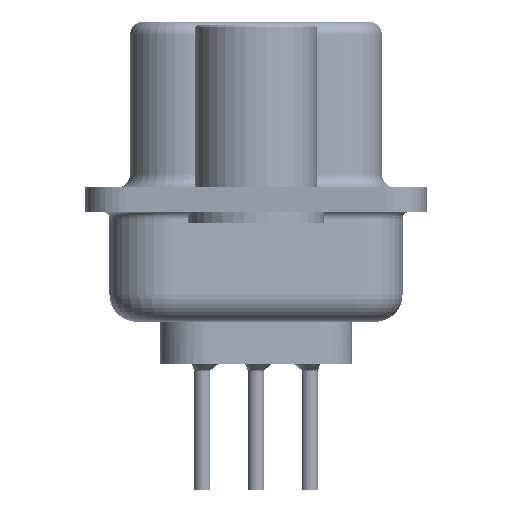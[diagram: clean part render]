
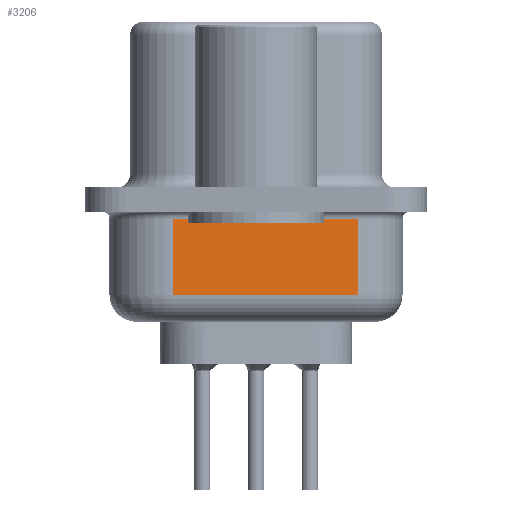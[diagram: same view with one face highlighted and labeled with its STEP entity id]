
A CAD part, left-side view. The second image highlights one B-rep face of the part: STEP entity #3206.
In plain terms, the highlighted planar face has unit normal (-0.985, -0.174, 0).
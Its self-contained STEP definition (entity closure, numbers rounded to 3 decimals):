
#273 = EDGE_CURVE ( 'NONE', #283, #12234, #12534, .T. ) ;
#283 = VERTEX_POINT ( 'NONE', #15796 ) ;
#637 = DIRECTION ( 'NONE',  ( -0.174, 0.985, 0. ) ) ;
#844 = DIRECTION ( 'NONE',  ( 0.174, -0.985, 0. ) ) ;
#3206 = ADVANCED_FACE ( 'NONE', ( #3270 ), #21578, .F. ) ;
#3270 = FACE_OUTER_BOUND ( 'NONE', #10184, .T. ) ;
#4048 = CARTESIAN_POINT ( 'NONE',  ( 3.13, 3.053, -0.7 ) ) ;
#5361 = EDGE_CURVE ( 'NONE', #12234, #35679, #33386, .T. ) ;
#8144 = VECTOR ( 'NONE', #844, 1000. ) ;
#9173 = CARTESIAN_POINT ( 'NONE',  ( 3.13, 3.053, -4.5 ) ) ;
#9586 = CARTESIAN_POINT ( 'NONE',  ( 3.13, 3.053, -3.5 ) ) ;
#10184 = EDGE_LOOP ( 'NONE', ( #37867, #31781, #35434, #33595 ) ) ;
#12234 = VERTEX_POINT ( 'NONE', #38557 ) ;
#12534 = LINE ( 'NONE', #36908, #39516 ) ;
#15191 = LINE ( 'NONE', #27587, #17185 ) ;
#15393 = DIRECTION ( 'NONE',  ( 0., 0., 1. ) ) ;
#15796 = CARTESIAN_POINT ( 'NONE',  ( 4.329, -3.747, -3.5 ) ) ;
#16301 = LINE ( 'NONE', #9586, #8144 ) ;
#17185 = VECTOR ( 'NONE', #39946, 1000. ) ;
#21578 = PLANE ( 'NONE',  #35993 ) ;
#23676 = EDGE_CURVE ( 'NONE', #25859, #283, #16301, .T. ) ;
#24268 = DIRECTION ( 'NONE',  ( -0.174, 0.985, 0. ) ) ;
#25720 = VECTOR ( 'NONE', #24268, 1000. ) ;
#25859 = VERTEX_POINT ( 'NONE', #36115 ) ;
#27587 = CARTESIAN_POINT ( 'NONE',  ( 3.13, 3.053, -4.5 ) ) ;
#27675 = DIRECTION ( 'NONE',  ( 0.985, 0.174, 0. ) ) ;
#30349 = CARTESIAN_POINT ( 'NONE',  ( 3.13, 3.053, -0.7 ) ) ;
#31781 = ORIENTED_EDGE ( 'NONE', *, *, #23676, .T. ) ;
#31963 = EDGE_CURVE ( 'NONE', #25859, #35679, #15191, .T. ) ;
#33386 = LINE ( 'NONE', #30349, #25720 ) ;
#33595 = ORIENTED_EDGE ( 'NONE', *, *, #5361, .T. ) ;
#35434 = ORIENTED_EDGE ( 'NONE', *, *, #273, .T. ) ;
#35679 = VERTEX_POINT ( 'NONE', #4048 ) ;
#35993 = AXIS2_PLACEMENT_3D ( 'NONE', #9173, #27675, #637 ) ;
#36115 = CARTESIAN_POINT ( 'NONE',  ( 3.13, 3.053, -3.5 ) ) ;
#36908 = CARTESIAN_POINT ( 'NONE',  ( 4.329, -3.747, -4.5 ) ) ;
#37867 = ORIENTED_EDGE ( 'NONE', *, *, #31963, .F. ) ;
#38557 = CARTESIAN_POINT ( 'NONE',  ( 4.329, -3.747, -0.7 ) ) ;
#39516 = VECTOR ( 'NONE', #15393, 1000. ) ;
#39946 = DIRECTION ( 'NONE',  ( 0., 0., 1. ) ) ;
